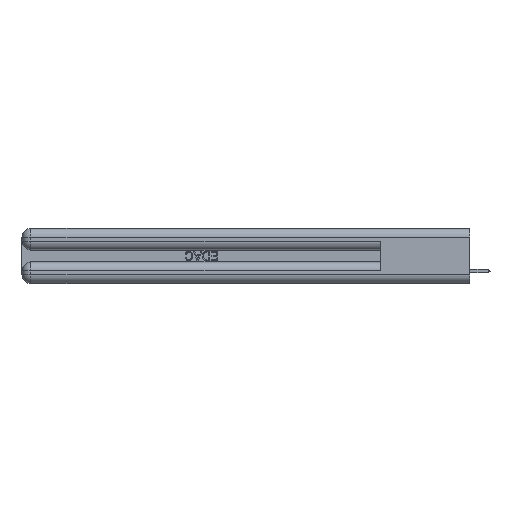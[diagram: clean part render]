
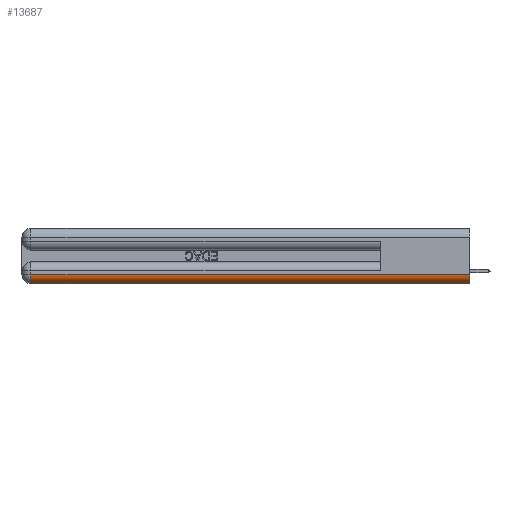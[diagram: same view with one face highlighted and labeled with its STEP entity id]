
A CAD part, left-side view. The second image highlights one B-rep face of the part: STEP entity #13687.
In plain terms, the highlighted cylindrical face has radius 1.524 mm (diameter 3.048 mm), a partial arc.
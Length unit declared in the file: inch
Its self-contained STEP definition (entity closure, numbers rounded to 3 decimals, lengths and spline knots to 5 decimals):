
#1912 = ORIENTED_EDGE ( 'NONE', *, *, #37115, .F. ) ;
#3940 = DIRECTION ( 'NONE',  ( 0., 0., 1. ) ) ;
#4764 = VECTOR ( 'NONE', #35413, 39.37008 ) ;
#5462 = VERTEX_POINT ( 'NONE', #31626 ) ;
#6550 = DIRECTION ( 'NONE',  ( 0., 0., 1. ) ) ;
#10002 = DIRECTION ( 'NONE',  ( 0., 1., 0. ) ) ;
#13687 = ADVANCED_FACE ( 'NONE', ( #29498 ), #49516, .T. ) ;
#14638 = CARTESIAN_POINT ( 'NONE',  ( 0.06, 3., 0. ) ) ;
#15160 = CARTESIAN_POINT ( 'NONE',  ( 0.06, 2.94, 0. ) ) ;
#16343 = CARTESIAN_POINT ( 'NONE',  ( 0.06, 0., 0.06 ) ) ;
#17416 = EDGE_CURVE ( 'NONE', #32025, #5462, #47904, .T. ) ;
#17863 = AXIS2_PLACEMENT_3D ( 'NONE', #38207, #10002, #42067 ) ;
#17937 = VERTEX_POINT ( 'NONE', #49991 ) ;
#18498 = VECTOR ( 'NONE', #43525, 39.37008 ) ;
#20175 = ORIENTED_EDGE ( 'NONE', *, *, #46667, .F. ) ;
#20491 = EDGE_LOOP ( 'NONE', ( #22382, #24212, #20175, #1912 ) ) ;
#22382 = ORIENTED_EDGE ( 'NONE', *, *, #29355, .F. ) ;
#24212 = ORIENTED_EDGE ( 'NONE', *, *, #17416, .F. ) ;
#25336 = CIRCLE ( 'NONE', #17863, 0.06 ) ;
#26378 = CIRCLE ( 'NONE', #44228, 0.06 ) ;
#29355 = EDGE_CURVE ( 'NONE', #5462, #17937, #26378, .T. ) ;
#29498 = FACE_OUTER_BOUND ( 'NONE', #20491, .T. ) ;
#31440 = AXIS2_PLACEMENT_3D ( 'NONE', #37892, #50360, #6550 ) ;
#31626 = CARTESIAN_POINT ( 'NONE',  ( 0., 0., 0.06 ) ) ;
#32025 = VERTEX_POINT ( 'NONE', #35319 ) ;
#33364 = VERTEX_POINT ( 'NONE', #15160 ) ;
#35319 = CARTESIAN_POINT ( 'NONE',  ( 0., 2.94, 0.06 ) ) ;
#35413 = DIRECTION ( 'NONE',  ( 0., -1., 0. ) ) ;
#37115 = EDGE_CURVE ( 'NONE', #17937, #33364, #49764, .T. ) ;
#37892 = CARTESIAN_POINT ( 'NONE',  ( 0.06, 0., 0.06 ) ) ;
#38207 = CARTESIAN_POINT ( 'NONE',  ( 0.06, 2.94, 0.06 ) ) ;
#38936 = CARTESIAN_POINT ( 'NONE',  ( 0., 0., 0.06 ) ) ;
#39155 = DIRECTION ( 'NONE',  ( 0., -1., 0. ) ) ;
#42067 = DIRECTION ( 'NONE',  ( 0., 0., 1. ) ) ;
#43525 = DIRECTION ( 'NONE',  ( 0., 1., 0. ) ) ;
#44228 = AXIS2_PLACEMENT_3D ( 'NONE', #16343, #39155, #3940 ) ;
#46667 = EDGE_CURVE ( 'NONE', #33364, #32025, #25336, .T. ) ;
#47904 = LINE ( 'NONE', #38936, #4764 ) ;
#49516 = CYLINDRICAL_SURFACE ( 'NONE', #31440, 0.06 ) ;
#49764 = LINE ( 'NONE', #14638, #18498 ) ;
#49991 = CARTESIAN_POINT ( 'NONE',  ( 0.06, 0., 0. ) ) ;
#50360 = DIRECTION ( 'NONE',  ( 0., 1., 0. ) ) ;
